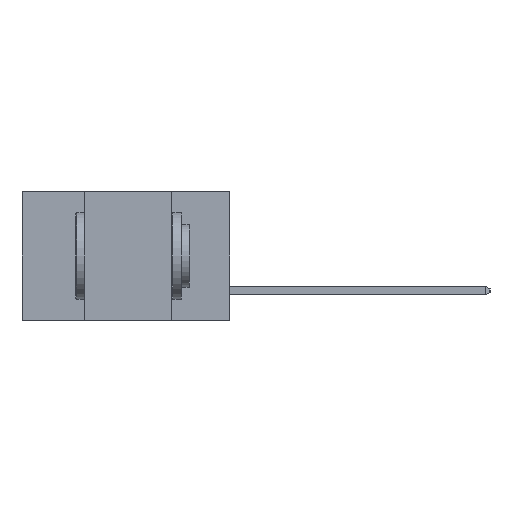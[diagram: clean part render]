
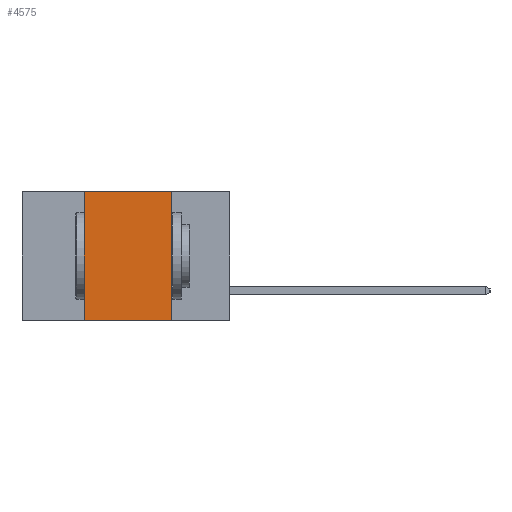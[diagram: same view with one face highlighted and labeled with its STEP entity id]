
A CAD part, left-side view. The second image highlights one B-rep face of the part: STEP entity #4575.
In plain terms, the highlighted planar face has unit normal (-1, 0, 0).
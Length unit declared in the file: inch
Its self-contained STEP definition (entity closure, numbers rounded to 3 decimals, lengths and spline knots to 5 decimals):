
#699 = CARTESIAN_POINT ( 'NONE',  ( 0., 0.17, -0.37 ) ) ;
#837 = EDGE_LOOP ( 'NONE', ( #2425, #1016, #5339, #2473 ) ) ;
#1016 = ORIENTED_EDGE ( 'NONE', *, *, #12566, .F. ) ;
#1052 = LINE ( 'NONE', #699, #4489 ) ;
#2256 = CARTESIAN_POINT ( 'NONE',  ( 0., 0.17, 0. ) ) ;
#2425 = ORIENTED_EDGE ( 'NONE', *, *, #16512, .F. ) ;
#2473 = ORIENTED_EDGE ( 'NONE', *, *, #4105, .T. ) ;
#2571 = VERTEX_POINT ( 'NONE', #2256 ) ;
#3106 = CARTESIAN_POINT ( 'NONE',  ( 0., 0.42, -0.37 ) ) ;
#3857 = CARTESIAN_POINT ( 'NONE',  ( 0., 0.17, -0.37 ) ) ;
#4105 = EDGE_CURVE ( 'NONE', #11627, #13283, #9726, .T. ) ;
#4489 = VECTOR ( 'NONE', #8588, 39.37008 ) ;
#4575 = ADVANCED_FACE ( 'NONE', ( #5602 ), #7023, .F. ) ;
#5112 = CARTESIAN_POINT ( 'NONE',  ( 0., 0.6, -0.37 ) ) ;
#5134 = DIRECTION ( 'NONE',  ( 0., -1., 0. ) ) ;
#5158 = DIRECTION ( 'NONE',  ( 0., -1., 0. ) ) ;
#5339 = ORIENTED_EDGE ( 'NONE', *, *, #7698, .F. ) ;
#5602 = FACE_OUTER_BOUND ( 'NONE', #837, .T. ) ;
#7002 = CARTESIAN_POINT ( 'NONE',  ( 0., 0.6, 0. ) ) ;
#7023 = PLANE ( 'NONE',  #14020 ) ;
#7103 = DIRECTION ( 'NONE',  ( 0., 0., -1. ) ) ;
#7106 = DIRECTION ( 'NONE',  ( 1., 0., 0. ) ) ;
#7698 = EDGE_CURVE ( 'NONE', #11627, #15120, #15595, .T. ) ;
#8331 = CARTESIAN_POINT ( 'NONE',  ( 0., 0.42, 0. ) ) ;
#8588 = DIRECTION ( 'NONE',  ( 0., 0., -1. ) ) ;
#9317 = VECTOR ( 'NONE', #5134, 39.37008 ) ;
#9726 = LINE ( 'NONE', #5112, #9317 ) ;
#10395 = CARTESIAN_POINT ( 'NONE',  ( 0., 0.6, 0. ) ) ;
#11624 = CARTESIAN_POINT ( 'NONE',  ( 0., 0.42, -0.37 ) ) ;
#11627 = VERTEX_POINT ( 'NONE', #3106 ) ;
#11682 = DIRECTION ( 'NONE',  ( 0., 0., 1. ) ) ;
#11823 = VECTOR ( 'NONE', #5158, 39.37008 ) ;
#12178 = VECTOR ( 'NONE', #11682, 39.37008 ) ;
#12566 = EDGE_CURVE ( 'NONE', #15120, #2571, #15263, .T. ) ;
#13283 = VERTEX_POINT ( 'NONE', #3857 ) ;
#14020 = AXIS2_PLACEMENT_3D ( 'NONE', #7002, #7106, #7103 ) ;
#15120 = VERTEX_POINT ( 'NONE', #8331 ) ;
#15263 = LINE ( 'NONE', #10395, #11823 ) ;
#15595 = LINE ( 'NONE', #11624, #12178 ) ;
#16512 = EDGE_CURVE ( 'NONE', #2571, #13283, #1052, .T. ) ;
